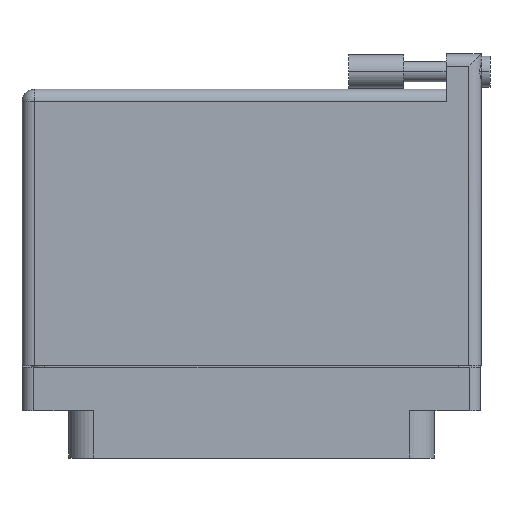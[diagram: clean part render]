
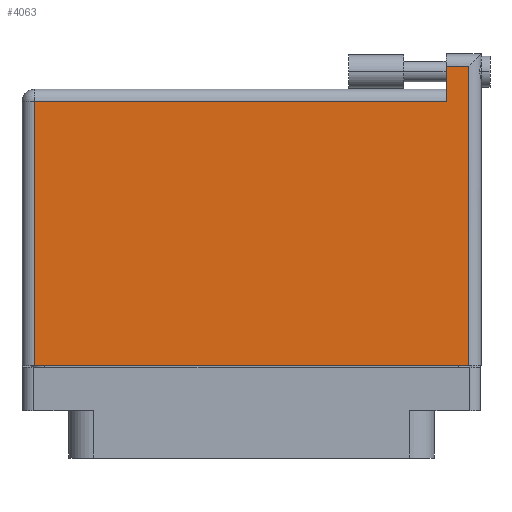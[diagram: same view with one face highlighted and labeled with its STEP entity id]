
A CAD part, front view. The second image highlights one B-rep face of the part: STEP entity #4063.
In plain terms, the highlighted face is planar.
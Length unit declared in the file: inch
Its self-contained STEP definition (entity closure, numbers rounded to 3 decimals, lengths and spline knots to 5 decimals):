
#585 = DIRECTION ( 'NONE',  ( 0., 1., 0. ) ) ;
#1238 = EDGE_LOOP ( 'NONE', ( #46321, #40590, #38981, #8521, #33269, #18162 ) ) ;
#1361 = AXIS2_PLACEMENT_3D ( 'NONE', #5099, #30624, #34664 ) ;
#2670 = CARTESIAN_POINT ( 'NONE',  ( -1.3, -0.1, 0.4495 ) ) ;
#2744 = DIRECTION ( 'NONE',  ( 0., -1., 0. ) ) ;
#3215 = CARTESIAN_POINT ( 'NONE',  ( 1.103, 1.396, 0.4495 ) ) ;
#4063 = ADVANCED_FACE ( 'NONE', ( #32552 ), #23097, .F. ) ;
#4105 = LINE ( 'NONE', #28297, #12746 ) ;
#4227 = CARTESIAN_POINT ( 'NONE',  ( -1.23, 1.396, 0.4495 ) ) ;
#5099 = CARTESIAN_POINT ( 'NONE',  ( -1.3, 1.466, 0.4495 ) ) ;
#7123 = DIRECTION ( 'NONE',  ( -1., 0., 0. ) ) ;
#7430 = VERTEX_POINT ( 'NONE', #3215 ) ;
#8059 = VECTOR ( 'NONE', #28070, 39.37008 ) ;
#8233 = CARTESIAN_POINT ( 'NONE',  ( -1.23, -0.1, 0.4495 ) ) ;
#8521 = ORIENTED_EDGE ( 'NONE', *, *, #20250, .T. ) ;
#8724 = LINE ( 'NONE', #9505, #28779 ) ;
#9505 = CARTESIAN_POINT ( 'NONE',  ( 1.103, 1.666, 0.4495 ) ) ;
#9656 = LINE ( 'NONE', #26773, #18310 ) ;
#11944 = VERTEX_POINT ( 'NONE', #39416 ) ;
#12746 = VECTOR ( 'NONE', #2744, 39.37008 ) ;
#13987 = CARTESIAN_POINT ( 'NONE',  ( 1.103, 1.596, 0.4495 ) ) ;
#14754 = VERTEX_POINT ( 'NONE', #13987 ) ;
#18162 = ORIENTED_EDGE ( 'NONE', *, *, #20227, .T. ) ;
#18310 = VECTOR ( 'NONE', #585, 39.37008 ) ;
#20227 = EDGE_CURVE ( 'NONE', #30673, #37625, #4105, .T. ) ;
#20250 = EDGE_CURVE ( 'NONE', #14754, #7430, #8724, .T. ) ;
#22237 = EDGE_CURVE ( 'NONE', #7430, #30673, #42560, .T. ) ;
#22487 = VECTOR ( 'NONE', #44005, 39.37008 ) ;
#23097 = PLANE ( 'NONE',  #1361 ) ;
#26773 = CARTESIAN_POINT ( 'NONE',  ( 1.23, 1.666, 0.4495 ) ) ;
#28070 = DIRECTION ( 'NONE',  ( 1., 0., 0. ) ) ;
#28297 = CARTESIAN_POINT ( 'NONE',  ( -1.23, -0.1, 0.4495 ) ) ;
#28779 = VECTOR ( 'NONE', #35224, 39.37008 ) ;
#30483 = EDGE_CURVE ( 'NONE', #36626, #14754, #35695, .T. ) ;
#30624 = DIRECTION ( 'NONE',  ( 0., 0., -1. ) ) ;
#30673 = VERTEX_POINT ( 'NONE', #4227 ) ;
#31904 = EDGE_CURVE ( 'NONE', #37625, #11944, #36814, .T. ) ;
#32552 = FACE_OUTER_BOUND ( 'NONE', #1238, .T. ) ;
#32795 = EDGE_CURVE ( 'NONE', #11944, #36626, #9656, .T. ) ;
#32805 = VECTOR ( 'NONE', #7123, 39.37008 ) ;
#33269 = ORIENTED_EDGE ( 'NONE', *, *, #22237, .T. ) ;
#34664 = DIRECTION ( 'NONE',  ( -1., 0., 0. ) ) ;
#35224 = DIRECTION ( 'NONE',  ( 0., -1., 0. ) ) ;
#35695 = LINE ( 'NONE', #43546, #32805 ) ;
#36594 = CARTESIAN_POINT ( 'NONE',  ( 1.23, 1.596, 0.4495 ) ) ;
#36626 = VERTEX_POINT ( 'NONE', #36594 ) ;
#36814 = LINE ( 'NONE', #2670, #8059 ) ;
#37625 = VERTEX_POINT ( 'NONE', #8233 ) ;
#38981 = ORIENTED_EDGE ( 'NONE', *, *, #30483, .T. ) ;
#39416 = CARTESIAN_POINT ( 'NONE',  ( 1.23, -0.1, 0.4495 ) ) ;
#40156 = CARTESIAN_POINT ( 'NONE',  ( -1.3, 1.396, 0.4495 ) ) ;
#40590 = ORIENTED_EDGE ( 'NONE', *, *, #32795, .T. ) ;
#42560 = LINE ( 'NONE', #40156, #22487 ) ;
#43546 = CARTESIAN_POINT ( 'NONE',  ( -1.3, 1.596, 0.4495 ) ) ;
#44005 = DIRECTION ( 'NONE',  ( -1., 0., 0. ) ) ;
#46321 = ORIENTED_EDGE ( 'NONE', *, *, #31904, .T. ) ;
